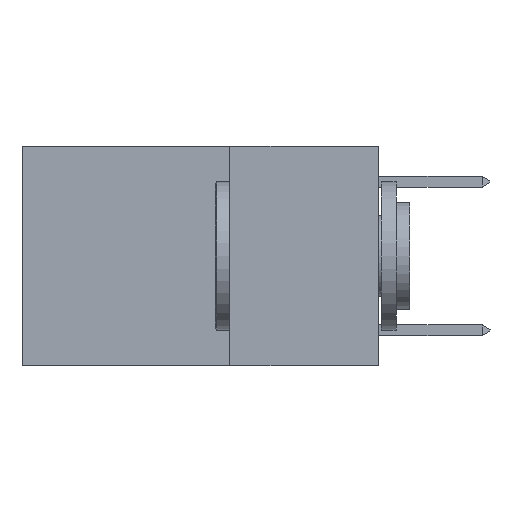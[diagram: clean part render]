
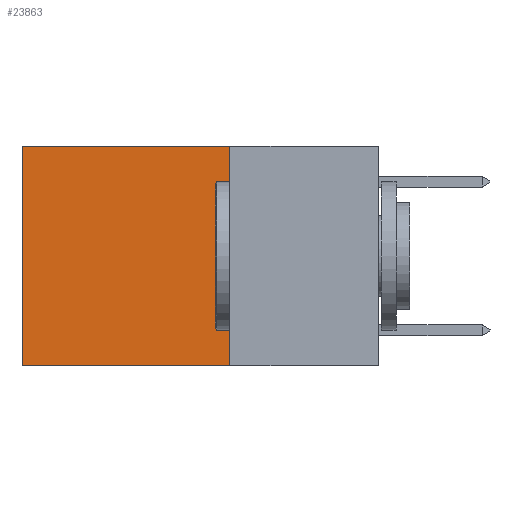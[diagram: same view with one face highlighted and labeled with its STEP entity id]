
A CAD part, left-side view. The second image highlights one B-rep face of the part: STEP entity #23863.
In plain terms, the highlighted planar face has unit normal (-1, 0, 0).
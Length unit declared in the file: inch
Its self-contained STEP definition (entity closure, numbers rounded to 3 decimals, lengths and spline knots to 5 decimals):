
#71 = LINE ( 'NONE', #2266, #15676 ) ;
#328 = CARTESIAN_POINT ( 'NONE',  ( 0.2625, 0.25, 0. ) ) ;
#581 = VERTEX_POINT ( 'NONE', #3247 ) ;
#1711 = CARTESIAN_POINT ( 'NONE',  ( 0.2625, 0.25, 0. ) ) ;
#1791 = AXIS2_PLACEMENT_3D ( 'NONE', #328, #8690, #1993 ) ;
#1993 = DIRECTION ( 'NONE',  ( 0., 0., -1. ) ) ;
#2043 = VERTEX_POINT ( 'NONE', #10227 ) ;
#2127 = FACE_OUTER_BOUND ( 'NONE', #17763, .T. ) ;
#2266 = CARTESIAN_POINT ( 'NONE',  ( 0.2625, 0.25, 0. ) ) ;
#2351 = VERTEX_POINT ( 'NONE', #15552 ) ;
#2463 = CARTESIAN_POINT ( 'NONE',  ( 0.2625, 0.25, -0.37 ) ) ;
#3247 = CARTESIAN_POINT ( 'NONE',  ( 0.2625, 0.25, 0. ) ) ;
#3441 = ORIENTED_EDGE ( 'NONE', *, *, #8498, .T. ) ;
#4638 = ORIENTED_EDGE ( 'NONE', *, *, #9507, .F. ) ;
#5288 = VERTEX_POINT ( 'NONE', #17162 ) ;
#5349 = ORIENTED_EDGE ( 'NONE', *, *, #14694, .F. ) ;
#6518 = VECTOR ( 'NONE', #11814, 39.37008 ) ;
#8498 = EDGE_CURVE ( 'NONE', #5288, #2043, #13603, .T. ) ;
#8690 = DIRECTION ( 'NONE',  ( 1., 0., 0. ) ) ;
#9507 = EDGE_CURVE ( 'NONE', #581, #2351, #71, .T. ) ;
#9516 = LINE ( 'NONE', #1711, #13268 ) ;
#10227 = CARTESIAN_POINT ( 'NONE',  ( 0.2625, 0.6, -0.37 ) ) ;
#10801 = DIRECTION ( 'NONE',  ( 0., 1., 0. ) ) ;
#11814 = DIRECTION ( 'NONE',  ( 0., 0., -1. ) ) ;
#12794 = PLANE ( 'NONE',  #1791 ) ;
#13268 = VECTOR ( 'NONE', #20070, 39.37008 ) ;
#13468 = CARTESIAN_POINT ( 'NONE',  ( 0.2625, 0.6, 0. ) ) ;
#13603 = LINE ( 'NONE', #13468, #6518 ) ;
#14694 = EDGE_CURVE ( 'NONE', #2351, #2043, #25326, .T. ) ;
#15552 = CARTESIAN_POINT ( 'NONE',  ( 0.2625, 0.25, -0.37 ) ) ;
#15676 = VECTOR ( 'NONE', #18980, 39.37008 ) ;
#17012 = EDGE_CURVE ( 'NONE', #581, #5288, #9516, .T. ) ;
#17162 = CARTESIAN_POINT ( 'NONE',  ( 0.2625, 0.6, 0. ) ) ;
#17763 = EDGE_LOOP ( 'NONE', ( #3441, #5349, #4638, #25444 ) ) ;
#18980 = DIRECTION ( 'NONE',  ( 0., 0., -1. ) ) ;
#20070 = DIRECTION ( 'NONE',  ( 0., 1., 0. ) ) ;
#22881 = VECTOR ( 'NONE', #10801, 39.37008 ) ;
#23863 = ADVANCED_FACE ( 'NONE', ( #2127 ), #12794, .F. ) ;
#25326 = LINE ( 'NONE', #2463, #22881 ) ;
#25444 = ORIENTED_EDGE ( 'NONE', *, *, #17012, .T. ) ;
